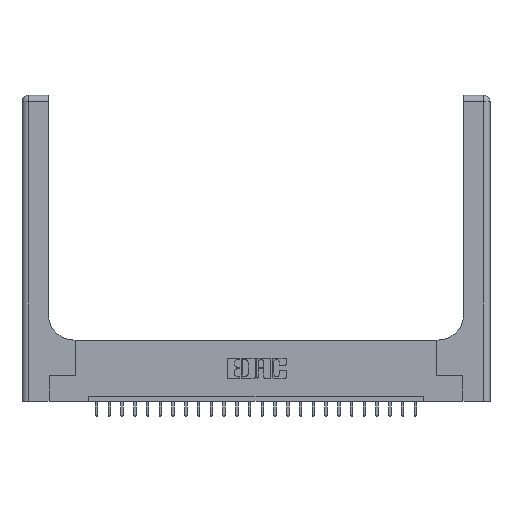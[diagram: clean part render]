
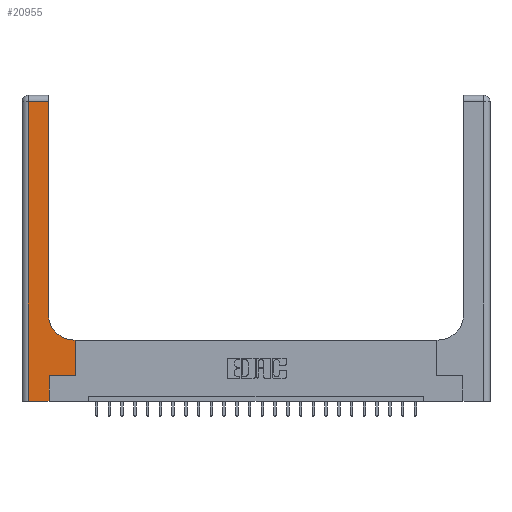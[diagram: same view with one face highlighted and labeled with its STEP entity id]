
A CAD part, top view. The second image highlights one B-rep face of the part: STEP entity #20955.
In plain terms, the highlighted planar face has unit normal (0, 0, 1).
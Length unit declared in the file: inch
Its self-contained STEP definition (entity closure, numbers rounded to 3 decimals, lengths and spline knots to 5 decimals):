
#263 = CARTESIAN_POINT ( 'NONE',  ( 0.528, 0.25, 0.37 ) ) ;
#614 = VECTOR ( 'NONE', #19707, 39.37008 ) ;
#971 = ORIENTED_EDGE ( 'NONE', *, *, #22217, .T. ) ;
#986 = LINE ( 'NONE', #6413, #9450 ) ;
#1242 = ORIENTED_EDGE ( 'NONE', *, *, #17019, .T. ) ;
#2240 = PLANE ( 'NONE',  #18913 ) ;
#2241 = AXIS2_PLACEMENT_3D ( 'NONE', #7886, #15190, #6142 ) ;
#2824 = CARTESIAN_POINT ( 'NONE',  ( 0.265, 0.25, 0.37 ) ) ;
#3140 = EDGE_CURVE ( 'NONE', #19784, #21377, #22454, .T. ) ;
#3541 = CARTESIAN_POINT ( 'NONE',  ( 0.265, 0.25, 0.37 ) ) ;
#3551 = LINE ( 'NONE', #2824, #19140 ) ;
#4072 = DIRECTION ( 'NONE',  ( 0., -1., 0. ) ) ;
#4830 = LINE ( 'NONE', #8903, #10217 ) ;
#4934 = CARTESIAN_POINT ( 'NONE',  ( 0., 2.94, 0.37 ) ) ;
#5122 = CARTESIAN_POINT ( 'NONE',  ( 0.265, 0., 0.37 ) ) ;
#5156 = DIRECTION ( 'NONE',  ( 0., 0., -1. ) ) ;
#5411 = LINE ( 'NONE', #12575, #614 ) ;
#5520 = VERTEX_POINT ( 'NONE', #263 ) ;
#5532 = EDGE_CURVE ( 'NONE', #13027, #19784, #19514, .T. ) ;
#5590 = CARTESIAN_POINT ( 'NONE',  ( 0.06, 2.94, 0.37 ) ) ;
#6142 = DIRECTION ( 'NONE',  ( 1., 0., 0. ) ) ;
#6162 = ORIENTED_EDGE ( 'NONE', *, *, #5532, .T. ) ;
#6413 = CARTESIAN_POINT ( 'NONE',  ( 0.26, 0.6, 0.37 ) ) ;
#6821 = CIRCLE ( 'NONE', #2241, 0.25 ) ;
#7548 = CARTESIAN_POINT ( 'NONE',  ( 0.26, 3., 0.37 ) ) ;
#7772 = VECTOR ( 'NONE', #14043, 39.37008 ) ;
#7878 = CARTESIAN_POINT ( 'NONE',  ( 0.06, 3., 0.37 ) ) ;
#7886 = CARTESIAN_POINT ( 'NONE',  ( 0.51, 0.85, 0.37 ) ) ;
#7975 = VECTOR ( 'NONE', #17469, 39.37008 ) ;
#8075 = FACE_OUTER_BOUND ( 'NONE', #22554, .T. ) ;
#8388 = VERTEX_POINT ( 'NONE', #19919 ) ;
#8903 = CARTESIAN_POINT ( 'NONE',  ( 0.265, 0., 0.37 ) ) ;
#9372 = DIRECTION ( 'NONE',  ( 0., 1., 0. ) ) ;
#9450 = VECTOR ( 'NONE', #19098, 39.37008 ) ;
#9657 = CARTESIAN_POINT ( 'NONE',  ( 0.26, 2.94, 0.37 ) ) ;
#10217 = VECTOR ( 'NONE', #19773, 39.37008 ) ;
#10735 = CARTESIAN_POINT ( 'NONE',  ( 0.26, 0.85, 0.37 ) ) ;
#10747 = VERTEX_POINT ( 'NONE', #5122 ) ;
#11623 = CARTESIAN_POINT ( 'NONE',  ( 0.528, 0.6, 0.37 ) ) ;
#12021 = VERTEX_POINT ( 'NONE', #11623 ) ;
#12166 = CARTESIAN_POINT ( 'NONE',  ( 0.06, 0., 0.37 ) ) ;
#12203 = DIRECTION ( 'NONE',  ( -1., 0., 0. ) ) ;
#12253 = EDGE_CURVE ( 'NONE', #8388, #13027, #6821, .T. ) ;
#12575 = CARTESIAN_POINT ( 'NONE',  ( 0., 0., 0.37 ) ) ;
#12613 = LINE ( 'NONE', #21248, #7772 ) ;
#13027 = VERTEX_POINT ( 'NONE', #10735 ) ;
#13551 = ORIENTED_EDGE ( 'NONE', *, *, #18796, .T. ) ;
#14002 = ORIENTED_EDGE ( 'NONE', *, *, #3140, .T. ) ;
#14043 = DIRECTION ( 'NONE',  ( 0., 1., 0. ) ) ;
#14891 = EDGE_CURVE ( 'NONE', #12021, #8388, #986, .T. ) ;
#15190 = DIRECTION ( 'NONE',  ( 0., 0., -1. ) ) ;
#15337 = DIRECTION ( 'NONE',  ( 1., 0., 0. ) ) ;
#16779 = ORIENTED_EDGE ( 'NONE', *, *, #12253, .T. ) ;
#17019 = EDGE_CURVE ( 'NONE', #10747, #21136, #4830, .T. ) ;
#17195 = ORIENTED_EDGE ( 'NONE', *, *, #19447, .T. ) ;
#17241 = VECTOR ( 'NONE', #9372, 39.37008 ) ;
#17469 = DIRECTION ( 'NONE',  ( -1., 0., 0. ) ) ;
#18484 = VECTOR ( 'NONE', #4072, 39.37008 ) ;
#18796 = EDGE_CURVE ( 'NONE', #21136, #5520, #3551, .T. ) ;
#18913 = AXIS2_PLACEMENT_3D ( 'NONE', #20075, #5156, #12203 ) ;
#19098 = DIRECTION ( 'NONE',  ( -1., 0., 0. ) ) ;
#19140 = VECTOR ( 'NONE', #15337, 39.37008 ) ;
#19447 = EDGE_CURVE ( 'NONE', #5520, #12021, #12613, .T. ) ;
#19514 = LINE ( 'NONE', #7548, #17241 ) ;
#19707 = DIRECTION ( 'NONE',  ( 1., 0., 0. ) ) ;
#19773 = DIRECTION ( 'NONE',  ( 0., 1., 0. ) ) ;
#19784 = VERTEX_POINT ( 'NONE', #9657 ) ;
#19919 = CARTESIAN_POINT ( 'NONE',  ( 0.51, 0.6, 0.37 ) ) ;
#19927 = LINE ( 'NONE', #7878, #18484 ) ;
#20075 = CARTESIAN_POINT ( 'NONE',  ( 0., 3., 0.37 ) ) ;
#20955 = ADVANCED_FACE ( 'NONE', ( #8075 ), #2240, .F. ) ;
#21136 = VERTEX_POINT ( 'NONE', #3541 ) ;
#21248 = CARTESIAN_POINT ( 'NONE',  ( 0.528, 0.25, 0.37 ) ) ;
#21377 = VERTEX_POINT ( 'NONE', #5590 ) ;
#22217 = EDGE_CURVE ( 'NONE', #21377, #23473, #19927, .T. ) ;
#22220 = ORIENTED_EDGE ( 'NONE', *, *, #22954, .T. ) ;
#22282 = ORIENTED_EDGE ( 'NONE', *, *, #14891, .T. ) ;
#22454 = LINE ( 'NONE', #4934, #7975 ) ;
#22554 = EDGE_LOOP ( 'NONE', ( #6162, #14002, #971, #22220, #1242, #13551, #17195, #22282, #16779 ) ) ;
#22954 = EDGE_CURVE ( 'NONE', #23473, #10747, #5411, .T. ) ;
#23473 = VERTEX_POINT ( 'NONE', #12166 ) ;
